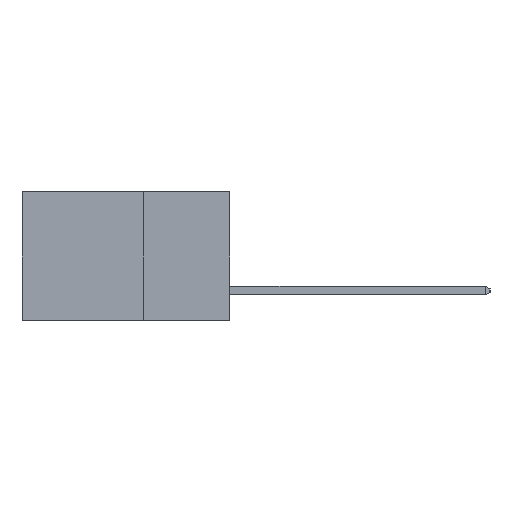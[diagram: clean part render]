
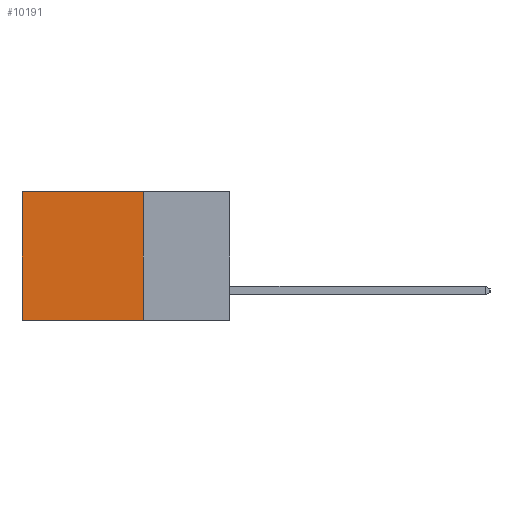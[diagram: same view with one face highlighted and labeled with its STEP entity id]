
A CAD part, left-side view. The second image highlights one B-rep face of the part: STEP entity #10191.
In plain terms, the highlighted planar face has unit normal (-1, 0, 0).
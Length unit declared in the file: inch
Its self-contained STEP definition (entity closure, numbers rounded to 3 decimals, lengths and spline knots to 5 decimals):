
#261 = EDGE_CURVE ( 'NONE', #773, #10164, #15796, .T. ) ;
#773 = VERTEX_POINT ( 'NONE', #14626 ) ;
#1216 = EDGE_LOOP ( 'NONE', ( #12474, #17121, #1360, #13748 ) ) ;
#1360 = ORIENTED_EDGE ( 'NONE', *, *, #3299, .F. ) ;
#3134 = VECTOR ( 'NONE', #5414, 39.37008 ) ;
#3299 = EDGE_CURVE ( 'NONE', #9654, #6368, #13133, .T. ) ;
#3503 = AXIS2_PLACEMENT_3D ( 'NONE', #15556, #7606, #16863 ) ;
#3667 = CARTESIAN_POINT ( 'NONE',  ( 0.2615, 0.6, -0.37 ) ) ;
#3936 = FACE_OUTER_BOUND ( 'NONE', #1216, .T. ) ;
#5048 = DIRECTION ( 'NONE',  ( 0., 0., -1. ) ) ;
#5414 = DIRECTION ( 'NONE',  ( 0., 0., -1. ) ) ;
#5661 = VECTOR ( 'NONE', #11778, 39.37008 ) ;
#6120 = CARTESIAN_POINT ( 'NONE',  ( 0.2615, 0.25, 0. ) ) ;
#6368 = VERTEX_POINT ( 'NONE', #13311 ) ;
#6793 = DIRECTION ( 'NONE',  ( 0., 1., 0. ) ) ;
#7542 = CARTESIAN_POINT ( 'NONE',  ( 0.2615, 0.6, -0.37 ) ) ;
#7606 = DIRECTION ( 'NONE',  ( 1., 0., 0. ) ) ;
#7689 = CARTESIAN_POINT ( 'NONE',  ( 0.2615, 0.25, 0. ) ) ;
#8754 = VECTOR ( 'NONE', #5048, 39.37008 ) ;
#9654 = VERTEX_POINT ( 'NONE', #6120 ) ;
#10164 = VERTEX_POINT ( 'NONE', #7542 ) ;
#10191 = ADVANCED_FACE ( 'NONE', ( #3936 ), #15501, .F. ) ;
#10465 = EDGE_CURVE ( 'NONE', #6368, #10164, #14088, .T. ) ;
#11778 = DIRECTION ( 'NONE',  ( 0., 1., 0. ) ) ;
#12212 = CARTESIAN_POINT ( 'NONE',  ( 0.2615, 0.25, -0.37 ) ) ;
#12474 = ORIENTED_EDGE ( 'NONE', *, *, #261, .T. ) ;
#13133 = LINE ( 'NONE', #13477, #3134 ) ;
#13311 = CARTESIAN_POINT ( 'NONE',  ( 0.2615, 0.25, -0.37 ) ) ;
#13477 = CARTESIAN_POINT ( 'NONE',  ( 0.2615, 0.25, -0.37 ) ) ;
#13748 = ORIENTED_EDGE ( 'NONE', *, *, #15960, .T. ) ;
#14088 = LINE ( 'NONE', #12212, #17122 ) ;
#14626 = CARTESIAN_POINT ( 'NONE',  ( 0.2615, 0.6, 0. ) ) ;
#15501 = PLANE ( 'NONE',  #3503 ) ;
#15556 = CARTESIAN_POINT ( 'NONE',  ( 0.2615, 0.25, -0.37 ) ) ;
#15796 = LINE ( 'NONE', #3667, #8754 ) ;
#15887 = LINE ( 'NONE', #7689, #5661 ) ;
#15960 = EDGE_CURVE ( 'NONE', #9654, #773, #15887, .T. ) ;
#16863 = DIRECTION ( 'NONE',  ( 0., 0., -1. ) ) ;
#17121 = ORIENTED_EDGE ( 'NONE', *, *, #10465, .F. ) ;
#17122 = VECTOR ( 'NONE', #6793, 39.37008 ) ;
